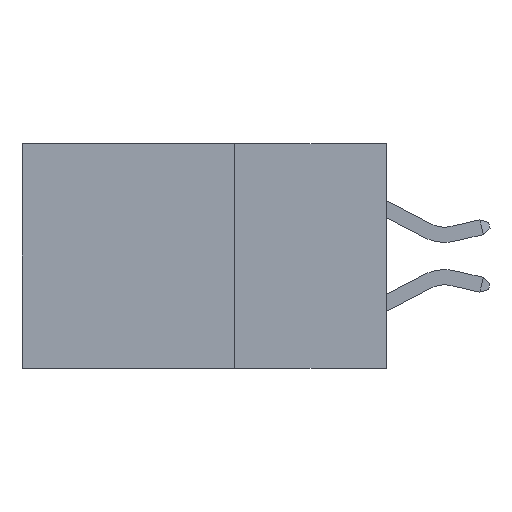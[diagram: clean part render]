
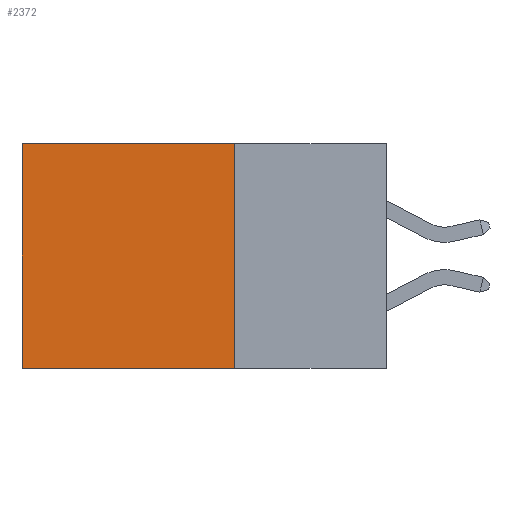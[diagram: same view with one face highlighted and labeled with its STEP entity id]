
A CAD part, left-side view. The second image highlights one B-rep face of the part: STEP entity #2372.
In plain terms, the highlighted planar face has unit normal (-1, 0, 0).
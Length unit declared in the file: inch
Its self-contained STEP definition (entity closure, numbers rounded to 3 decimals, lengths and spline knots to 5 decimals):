
#31 = LINE ( 'NONE', #16780, #9741 ) ;
#354 = CARTESIAN_POINT ( 'NONE',  ( 0.298, 0.6, 0. ) ) ;
#1036 = DIRECTION ( 'NONE',  ( 0., 0., -1. ) ) ;
#1725 = ORIENTED_EDGE ( 'NONE', *, *, #17398, .T. ) ;
#2271 = EDGE_LOOP ( 'NONE', ( #1725, #8200, #19068, #12691 ) ) ;
#2372 = ADVANCED_FACE ( 'NONE', ( #17617 ), #25928, .F. ) ;
#2738 = VECTOR ( 'NONE', #4855, 39.37008 ) ;
#3439 = VERTEX_POINT ( 'NONE', #354 ) ;
#4157 = VERTEX_POINT ( 'NONE', #6743 ) ;
#4379 = VERTEX_POINT ( 'NONE', #13681 ) ;
#4855 = DIRECTION ( 'NONE',  ( 0., 0., -1. ) ) ;
#6743 = CARTESIAN_POINT ( 'NONE',  ( 0.298, 0.25, -0.37 ) ) ;
#8200 = ORIENTED_EDGE ( 'NONE', *, *, #25120, .F. ) ;
#8238 = LINE ( 'NONE', #16926, #2738 ) ;
#9102 = CARTESIAN_POINT ( 'NONE',  ( 0.298, 0.25, 0. ) ) ;
#9573 = LINE ( 'NONE', #21626, #19395 ) ;
#9741 = VECTOR ( 'NONE', #18867, 39.37008 ) ;
#10998 = VERTEX_POINT ( 'NONE', #13382 ) ;
#11213 = AXIS2_PLACEMENT_3D ( 'NONE', #9102, #13496, #1036 ) ;
#12067 = CARTESIAN_POINT ( 'NONE',  ( 0.298, 0.25, 0. ) ) ;
#12691 = ORIENTED_EDGE ( 'NONE', *, *, #13095, .T. ) ;
#13095 = EDGE_CURVE ( 'NONE', #10998, #3439, #9573, .T. ) ;
#13362 = DIRECTION ( 'NONE',  ( 0., 1., 0. ) ) ;
#13382 = CARTESIAN_POINT ( 'NONE',  ( 0.298, 0.25, 0. ) ) ;
#13496 = DIRECTION ( 'NONE',  ( 1., 0., 0. ) ) ;
#13681 = CARTESIAN_POINT ( 'NONE',  ( 0.298, 0.6, -0.37 ) ) ;
#16136 = VECTOR ( 'NONE', #26587, 39.37008 ) ;
#16780 = CARTESIAN_POINT ( 'NONE',  ( 0.298, 0.25, -0.37 ) ) ;
#16806 = LINE ( 'NONE', #12067, #16136 ) ;
#16926 = CARTESIAN_POINT ( 'NONE',  ( 0.298, 0.6, 0. ) ) ;
#17398 = EDGE_CURVE ( 'NONE', #3439, #4379, #8238, .T. ) ;
#17617 = FACE_OUTER_BOUND ( 'NONE', #2271, .T. ) ;
#18867 = DIRECTION ( 'NONE',  ( 0., 1., 0. ) ) ;
#19068 = ORIENTED_EDGE ( 'NONE', *, *, #21854, .F. ) ;
#19395 = VECTOR ( 'NONE', #13362, 39.37008 ) ;
#21626 = CARTESIAN_POINT ( 'NONE',  ( 0.298, 0.25, 0. ) ) ;
#21854 = EDGE_CURVE ( 'NONE', #10998, #4157, #16806, .T. ) ;
#25120 = EDGE_CURVE ( 'NONE', #4157, #4379, #31, .T. ) ;
#25928 = PLANE ( 'NONE',  #11213 ) ;
#26587 = DIRECTION ( 'NONE',  ( 0., 0., -1. ) ) ;
